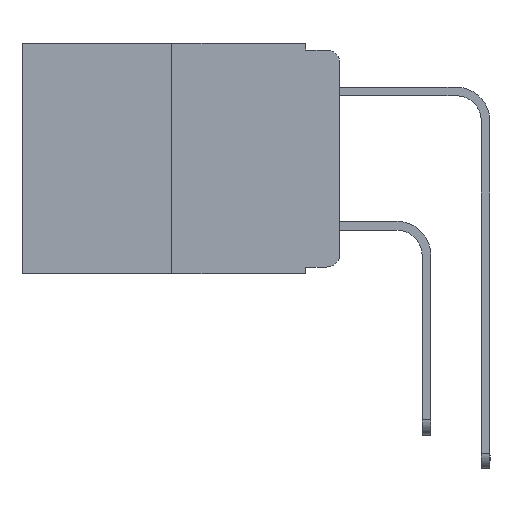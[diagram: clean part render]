
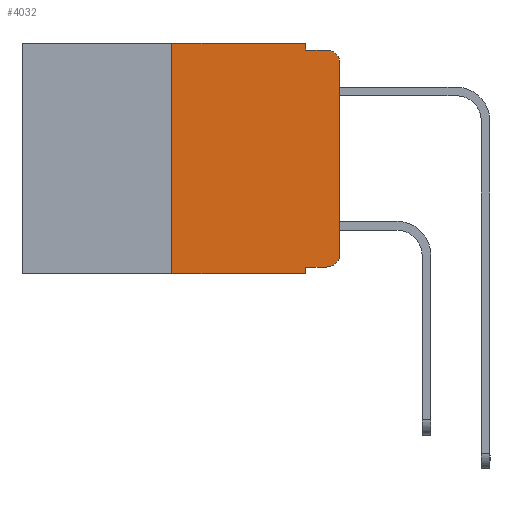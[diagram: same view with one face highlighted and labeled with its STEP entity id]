
A CAD part, left-side view. The second image highlights one B-rep face of the part: STEP entity #4032.
In plain terms, the highlighted planar face has unit normal (-1, 0, 0).
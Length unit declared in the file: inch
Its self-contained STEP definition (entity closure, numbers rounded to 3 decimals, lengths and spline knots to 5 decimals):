
#146 = ORIENTED_EDGE ( 'NONE', *, *, #9566, .F. ) ;
#1124 = CARTESIAN_POINT ( 'NONE',  ( 0., 0.051, -0.01 ) ) ;
#1491 = DIRECTION ( 'NONE',  ( 0., -1., 0. ) ) ;
#1694 = VERTEX_POINT ( 'NONE', #4479 ) ;
#1925 = VERTEX_POINT ( 'NONE', #1994 ) ;
#1994 = CARTESIAN_POINT ( 'NONE',  ( 0., 0.02, -0.333 ) ) ;
#2208 = CARTESIAN_POINT ( 'NONE',  ( 0., 0.02, -0.313 ) ) ;
#2252 = DIRECTION ( 'NONE',  ( 0., 0., -1. ) ) ;
#2640 = VECTOR ( 'NONE', #9791, 39.37008 ) ;
#2684 = ORIENTED_EDGE ( 'NONE', *, *, #13915, .T. ) ;
#2749 = ORIENTED_EDGE ( 'NONE', *, *, #4276, .F. ) ;
#3020 = EDGE_CURVE ( 'NONE', #19896, #12407, #23629, .T. ) ;
#3208 = LINE ( 'NONE', #1124, #19518 ) ;
#3529 = PLANE ( 'NONE',  #9523 ) ;
#3914 = DIRECTION ( 'NONE',  ( 0., 0., 1. ) ) ;
#4025 = LINE ( 'NONE', #7594, #2640 ) ;
#4032 = ADVANCED_FACE ( 'NONE', ( #20333 ), #3529, .F. ) ;
#4044 = CARTESIAN_POINT ( 'NONE',  ( 0., 0.25, -0.343 ) ) ;
#4276 = EDGE_CURVE ( 'NONE', #17094, #14646, #10250, .T. ) ;
#4479 = CARTESIAN_POINT ( 'NONE',  ( 0., 0.051, -0.343 ) ) ;
#5495 = DIRECTION ( 'NONE',  ( 0., 0., -1. ) ) ;
#5770 = EDGE_CURVE ( 'NONE', #21462, #1694, #18939, .T. ) ;
#6203 = CARTESIAN_POINT ( 'NONE',  ( 0., 0., -0.313 ) ) ;
#6328 = CARTESIAN_POINT ( 'NONE',  ( 0., 0.051, 0. ) ) ;
#6413 = VECTOR ( 'NONE', #2252, 39.37008 ) ;
#6594 = VERTEX_POINT ( 'NONE', #4044 ) ;
#7285 = CARTESIAN_POINT ( 'NONE',  ( 0., 0.051, -0.01 ) ) ;
#7423 = CIRCLE ( 'NONE', #21156, 0.02 ) ;
#7594 = CARTESIAN_POINT ( 'NONE',  ( 0., 0.051, 0. ) ) ;
#7864 = DIRECTION ( 'NONE',  ( -1., 0., 0. ) ) ;
#8744 = CARTESIAN_POINT ( 'NONE',  ( 0., 0.051, -0.333 ) ) ;
#9523 = AXIS2_PLACEMENT_3D ( 'NONE', #19973, #16657, #5495 ) ;
#9566 = EDGE_CURVE ( 'NONE', #14646, #18808, #4025, .T. ) ;
#9782 = VECTOR ( 'NONE', #23748, 39.37008 ) ;
#9791 = DIRECTION ( 'NONE',  ( 0., 0., -1. ) ) ;
#10139 = ORIENTED_EDGE ( 'NONE', *, *, #20451, .T. ) ;
#10250 = LINE ( 'NONE', #17504, #12790 ) ;
#10580 = LINE ( 'NONE', #8744, #18426 ) ;
#11004 = ORIENTED_EDGE ( 'NONE', *, *, #13837, .T. ) ;
#11228 = CARTESIAN_POINT ( 'NONE',  ( 0., 0.051, 0. ) ) ;
#11362 = ORIENTED_EDGE ( 'NONE', *, *, #19234, .F. ) ;
#11413 = CARTESIAN_POINT ( 'NONE',  ( 0., 0.25, 0. ) ) ;
#11646 = CIRCLE ( 'NONE', #13217, 0.02 ) ;
#12294 = CARTESIAN_POINT ( 'NONE',  ( 0., 0., -0.03 ) ) ;
#12323 = LINE ( 'NONE', #16089, #21546 ) ;
#12407 = VERTEX_POINT ( 'NONE', #12294 ) ;
#12790 = VECTOR ( 'NONE', #17627, 39.37008 ) ;
#12866 = CARTESIAN_POINT ( 'NONE',  ( 0., 0.051, -0.333 ) ) ;
#13217 = AXIS2_PLACEMENT_3D ( 'NONE', #2208, #7864, #13505 ) ;
#13497 = ORIENTED_EDGE ( 'NONE', *, *, #21127, .F. ) ;
#13505 = DIRECTION ( 'NONE',  ( 0., 0., -1. ) ) ;
#13837 = EDGE_CURVE ( 'NONE', #6594, #1694, #12323, .T. ) ;
#13915 = EDGE_CURVE ( 'NONE', #21462, #1925, #10580, .T. ) ;
#14646 = VERTEX_POINT ( 'NONE', #6328 ) ;
#14656 = CARTESIAN_POINT ( 'NONE',  ( 0., 0., 0. ) ) ;
#15117 = EDGE_LOOP ( 'NONE', ( #15539, #10139, #11362, #146, #2749, #13497, #11004, #22521, #2684, #21801 ) ) ;
#15214 = VECTOR ( 'NONE', #3914, 39.37008 ) ;
#15539 = ORIENTED_EDGE ( 'NONE', *, *, #3020, .T. ) ;
#15734 = VERTEX_POINT ( 'NONE', #23758 ) ;
#16089 = CARTESIAN_POINT ( 'NONE',  ( 0., 0.473, -0.343 ) ) ;
#16217 = DIRECTION ( 'NONE',  ( 0., -1., 0. ) ) ;
#16657 = DIRECTION ( 'NONE',  ( 1., 0., 0. ) ) ;
#17094 = VERTEX_POINT ( 'NONE', #22044 ) ;
#17504 = CARTESIAN_POINT ( 'NONE',  ( 0., 0.473, 0. ) ) ;
#17627 = DIRECTION ( 'NONE',  ( 0., -1., 0. ) ) ;
#17832 = DIRECTION ( 'NONE',  ( -1., 0., 0. ) ) ;
#18217 = EDGE_CURVE ( 'NONE', #1925, #19896, #11646, .T. ) ;
#18426 = VECTOR ( 'NONE', #16217, 39.37008 ) ;
#18808 = VERTEX_POINT ( 'NONE', #7285 ) ;
#18939 = LINE ( 'NONE', #11228, #6413 ) ;
#19234 = EDGE_CURVE ( 'NONE', #18808, #15734, #3208, .T. ) ;
#19518 = VECTOR ( 'NONE', #1491, 39.37008 ) ;
#19787 = DIRECTION ( 'NONE',  ( 0., -1., 0. ) ) ;
#19896 = VERTEX_POINT ( 'NONE', #6203 ) ;
#19973 = CARTESIAN_POINT ( 'NONE',  ( 0., 0.473, 0. ) ) ;
#20333 = FACE_OUTER_BOUND ( 'NONE', #15117, .T. ) ;
#20451 = EDGE_CURVE ( 'NONE', #12407, #15734, #7423, .T. ) ;
#20732 = LINE ( 'NONE', #11413, #15214 ) ;
#21127 = EDGE_CURVE ( 'NONE', #6594, #17094, #20732, .T. ) ;
#21156 = AXIS2_PLACEMENT_3D ( 'NONE', #22989, #17832, #21279 ) ;
#21279 = DIRECTION ( 'NONE',  ( 0., 0., -1. ) ) ;
#21462 = VERTEX_POINT ( 'NONE', #12866 ) ;
#21546 = VECTOR ( 'NONE', #19787, 39.37008 ) ;
#21801 = ORIENTED_EDGE ( 'NONE', *, *, #18217, .T. ) ;
#22044 = CARTESIAN_POINT ( 'NONE',  ( 0., 0.25, 0. ) ) ;
#22521 = ORIENTED_EDGE ( 'NONE', *, *, #5770, .F. ) ;
#22989 = CARTESIAN_POINT ( 'NONE',  ( 0., 0.02, -0.03 ) ) ;
#23629 = LINE ( 'NONE', #14656, #9782 ) ;
#23748 = DIRECTION ( 'NONE',  ( 0., 0., 1. ) ) ;
#23758 = CARTESIAN_POINT ( 'NONE',  ( 0., 0.02, -0.01 ) ) ;
